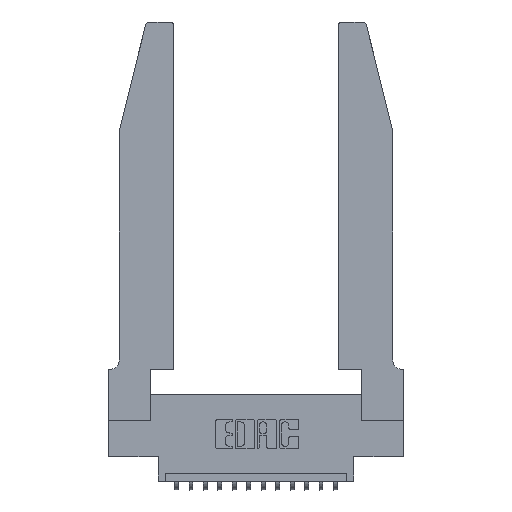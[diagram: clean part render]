
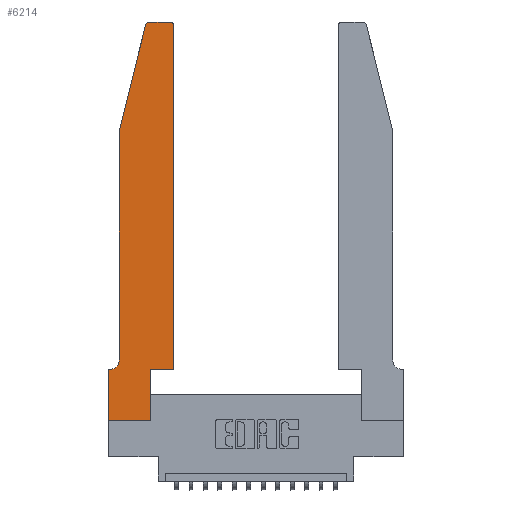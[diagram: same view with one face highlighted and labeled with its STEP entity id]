
A CAD part, top view. The second image highlights one B-rep face of the part: STEP entity #6214.
In plain terms, the highlighted planar face has unit normal (0, 0, 1).
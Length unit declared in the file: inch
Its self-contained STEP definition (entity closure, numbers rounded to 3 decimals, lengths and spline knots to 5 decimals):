
#61 = EDGE_CURVE ( 'NONE', #11342, #9079, #329, .T. ) ;
#120 = ORIENTED_EDGE ( 'NONE', *, *, #5008, .T. ) ;
#272 = CARTESIAN_POINT ( 'NONE',  ( 0.4505, 0.35, 0.37 ) ) ;
#329 = LINE ( 'NONE', #8984, #14064 ) ;
#379 = VECTOR ( 'NONE', #16272, 39.37008 ) ;
#450 = ORIENTED_EDGE ( 'NONE', *, *, #13431, .T. ) ;
#614 = VERTEX_POINT ( 'NONE', #12618 ) ;
#872 = VECTOR ( 'NONE', #7005, 39.37008 ) ;
#897 = DIRECTION ( 'NONE',  ( 1., 0., 0. ) ) ;
#921 = VERTEX_POINT ( 'NONE', #10727 ) ;
#960 = DIRECTION ( 'NONE',  ( -1., 0., 0. ) ) ;
#1064 = CARTESIAN_POINT ( 'NONE',  ( 0., 0.35, 0.37 ) ) ;
#1074 = LINE ( 'NONE', #6640, #4357 ) ;
#1239 = VERTEX_POINT ( 'NONE', #15503 ) ;
#1976 = ORIENTED_EDGE ( 'NONE', *, *, #9250, .T. ) ;
#2089 = EDGE_CURVE ( 'NONE', #614, #17835, #17681, .T. ) ;
#2260 = VERTEX_POINT ( 'NONE', #14649 ) ;
#2838 = ORIENTED_EDGE ( 'NONE', *, *, #4856, .T. ) ;
#3098 = DIRECTION ( 'NONE',  ( 0., 1., 0. ) ) ;
#3355 = CARTESIAN_POINT ( 'NONE',  ( 0., 0.35, 0.37 ) ) ;
#3916 = CARTESIAN_POINT ( 'NONE',  ( 0., 0., 0.37 ) ) ;
#4357 = VECTOR ( 'NONE', #960, 39.37008 ) ;
#4706 = CARTESIAN_POINT ( 'NONE',  ( 0., 0., 0.37 ) ) ;
#4856 = EDGE_CURVE ( 'NONE', #17835, #6693, #14357, .T. ) ;
#4941 = CARTESIAN_POINT ( 'NONE',  ( 0.4505, 0.35, 0.37 ) ) ;
#4943 = FACE_OUTER_BOUND ( 'NONE', #14584, .T. ) ;
#4960 = CARTESIAN_POINT ( 'NONE',  ( 0.0755, 2., 0.37 ) ) ;
#5008 = EDGE_CURVE ( 'NONE', #6693, #14874, #12650, .T. ) ;
#5028 = LINE ( 'NONE', #3916, #872 ) ;
#5312 = ORIENTED_EDGE ( 'NONE', *, *, #2089, .T. ) ;
#5401 = CIRCLE ( 'NONE', #8551, 0.07 ) ;
#5494 = LINE ( 'NONE', #8026, #13593 ) ;
#5756 = ORIENTED_EDGE ( 'NONE', *, *, #11753, .T. ) ;
#5767 = LINE ( 'NONE', #272, #12351 ) ;
#6104 = VERTEX_POINT ( 'NONE', #3355 ) ;
#6214 = ADVANCED_FACE ( 'NONE', ( #4943 ), #6686, .T. ) ;
#6287 = CARTESIAN_POINT ( 'NONE',  ( 0.2865, 0., 0.37 ) ) ;
#6532 = CARTESIAN_POINT ( 'NONE',  ( 0.2865, 0.35, 0.37 ) ) ;
#6640 = CARTESIAN_POINT ( 'NONE',  ( 0.2605, 2.75, 0.37 ) ) ;
#6686 = PLANE ( 'NONE',  #8976 ) ;
#6693 = VERTEX_POINT ( 'NONE', #4960 ) ;
#7005 = DIRECTION ( 'NONE',  ( 1., 0., 0. ) ) ;
#7028 = DIRECTION ( 'NONE',  ( 0., -1., 0. ) ) ;
#7064 = DIRECTION ( 'NONE',  ( -0.239, -0.971, 0. ) ) ;
#7146 = EDGE_CURVE ( 'NONE', #2260, #1239, #11475, .T. ) ;
#7268 = CARTESIAN_POINT ( 'NONE',  ( 0., 0., 0.37 ) ) ;
#7316 = EDGE_CURVE ( 'NONE', #9079, #2260, #5767, .T. ) ;
#7465 = CARTESIAN_POINT ( 'NONE',  ( 0.2865, 0.35, 0.37 ) ) ;
#7874 = DIRECTION ( 'NONE',  ( 0., 0., 1. ) ) ;
#8026 = CARTESIAN_POINT ( 'NONE',  ( 0.0755, 0.35, 0.37 ) ) ;
#8208 = CARTESIAN_POINT ( 'NONE',  ( 0.0755, 0.42, 0.37 ) ) ;
#8551 = AXIS2_PLACEMENT_3D ( 'NONE', #9516, #10919, #13685 ) ;
#8727 = EDGE_CURVE ( 'NONE', #6104, #14154, #10349, .T. ) ;
#8828 = ORIENTED_EDGE ( 'NONE', *, *, #7146, .T. ) ;
#8935 = ORIENTED_EDGE ( 'NONE', *, *, #7316, .T. ) ;
#8976 = AXIS2_PLACEMENT_3D ( 'NONE', #1064, #13578, #16324 ) ;
#8984 = CARTESIAN_POINT ( 'NONE',  ( 0.4505, 0.35, 0.37 ) ) ;
#9079 = VERTEX_POINT ( 'NONE', #4941 ) ;
#9250 = EDGE_CURVE ( 'NONE', #14154, #14604, #5028, .T. ) ;
#9293 = CARTESIAN_POINT ( 'NONE',  ( 0.0755, 2., 0.37 ) ) ;
#9516 = CARTESIAN_POINT ( 'NONE',  ( 0.0055, 0.42, 0.37 ) ) ;
#9804 = CARTESIAN_POINT ( 'NONE',  ( 0.0755, 2., 0.37 ) ) ;
#10017 = ORIENTED_EDGE ( 'NONE', *, *, #61, .T. ) ;
#10030 = DIRECTION ( 'NONE',  ( 0., 0., 1. ) ) ;
#10231 = ORIENTED_EDGE ( 'NONE', *, *, #8727, .T. ) ;
#10349 = LINE ( 'NONE', #7268, #14211 ) ;
#10407 = AXIS2_PLACEMENT_3D ( 'NONE', #14610, #7874, #897 ) ;
#10702 = VECTOR ( 'NONE', #7064, 39.37008 ) ;
#10712 = CARTESIAN_POINT ( 'NONE',  ( 0.25487, 2.72718, 0.37 ) ) ;
#10727 = CARTESIAN_POINT ( 'NONE',  ( 0.0055, 0.35, 0.37 ) ) ;
#10919 = DIRECTION ( 'NONE',  ( 0., 0., -1. ) ) ;
#10979 = DIRECTION ( 'NONE',  ( -1., 0., 0. ) ) ;
#11342 = VERTEX_POINT ( 'NONE', #7465 ) ;
#11475 = CIRCLE ( 'NONE', #10407, 0.03 ) ;
#11584 = ORIENTED_EDGE ( 'NONE', *, *, #16454, .T. ) ;
#11753 = EDGE_CURVE ( 'NONE', #14604, #11342, #15626, .T. ) ;
#11781 = DIRECTION ( 'NONE',  ( 1., 0., 0. ) ) ;
#12351 = VECTOR ( 'NONE', #3098, 39.37008 ) ;
#12566 = DIRECTION ( 'NONE',  ( 0., -1., 0. ) ) ;
#12618 = CARTESIAN_POINT ( 'NONE',  ( 0.284, 2.75, 0.37 ) ) ;
#12650 = LINE ( 'NONE', #9293, #15857 ) ;
#13431 = EDGE_CURVE ( 'NONE', #14874, #921, #5401, .T. ) ;
#13578 = DIRECTION ( 'NONE',  ( 0., 0., 1. ) ) ;
#13593 = VECTOR ( 'NONE', #10979, 39.37008 ) ;
#13685 = DIRECTION ( 'NONE',  ( -1., 0., 0. ) ) ;
#13766 = ORIENTED_EDGE ( 'NONE', *, *, #14849, .T. ) ;
#14064 = VECTOR ( 'NONE', #11781, 39.37008 ) ;
#14154 = VERTEX_POINT ( 'NONE', #4706 ) ;
#14211 = VECTOR ( 'NONE', #7028, 39.37008 ) ;
#14357 = LINE ( 'NONE', #9804, #10702 ) ;
#14584 = EDGE_LOOP ( 'NONE', ( #11584, #5312, #2838, #120, #450, #13766, #10231, #1976, #5756, #10017, #8935, #8828 ) ) ;
#14604 = VERTEX_POINT ( 'NONE', #6287 ) ;
#14610 = CARTESIAN_POINT ( 'NONE',  ( 0.4205, 2.72, 0.37 ) ) ;
#14649 = CARTESIAN_POINT ( 'NONE',  ( 0.4505, 2.72, 0.37 ) ) ;
#14849 = EDGE_CURVE ( 'NONE', #921, #6104, #5494, .T. ) ;
#14874 = VERTEX_POINT ( 'NONE', #8208 ) ;
#14967 = AXIS2_PLACEMENT_3D ( 'NONE', #15682, #10030, #17030 ) ;
#15503 = CARTESIAN_POINT ( 'NONE',  ( 0.4205, 2.75, 0.37 ) ) ;
#15626 = LINE ( 'NONE', #6532, #379 ) ;
#15682 = CARTESIAN_POINT ( 'NONE',  ( 0.284, 2.72, 0.37 ) ) ;
#15857 = VECTOR ( 'NONE', #12566, 39.37008 ) ;
#16272 = DIRECTION ( 'NONE',  ( 0., 1., 0. ) ) ;
#16324 = DIRECTION ( 'NONE',  ( 1., 0., 0. ) ) ;
#16454 = EDGE_CURVE ( 'NONE', #1239, #614, #1074, .T. ) ;
#17030 = DIRECTION ( 'NONE',  ( 1., 0., 0. ) ) ;
#17681 = CIRCLE ( 'NONE', #14967, 0.03 ) ;
#17835 = VERTEX_POINT ( 'NONE', #10712 ) ;
